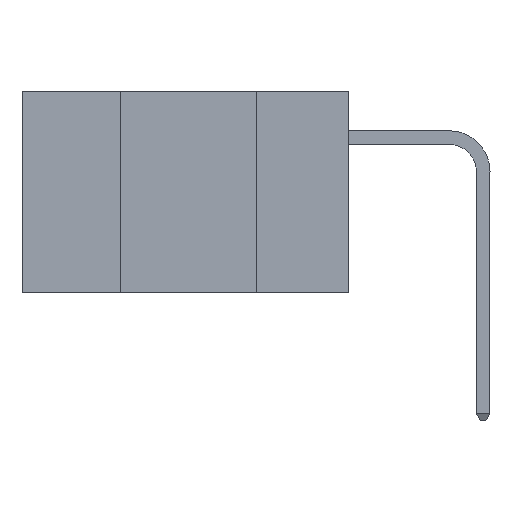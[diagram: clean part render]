
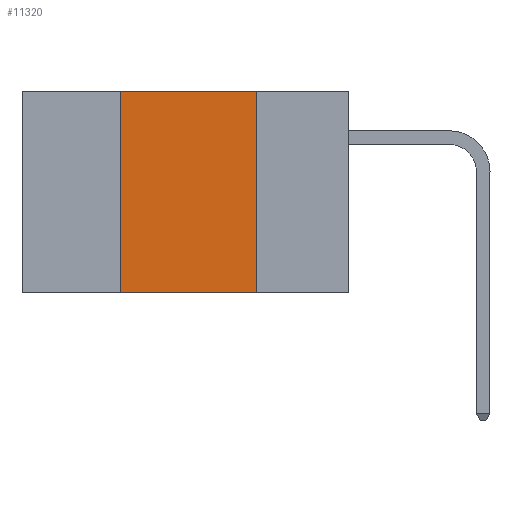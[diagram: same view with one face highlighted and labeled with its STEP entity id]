
A CAD part, left-side view. The second image highlights one B-rep face of the part: STEP entity #11320.
In plain terms, the highlighted planar face has unit normal (-1, 0, 0).
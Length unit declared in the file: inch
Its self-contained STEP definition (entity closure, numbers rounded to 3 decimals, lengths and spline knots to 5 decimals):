
#238 = ORIENTED_EDGE ( 'NONE', *, *, #440, .F. ) ;
#440 = EDGE_CURVE ( 'NONE', #15428, #15209, #568, .T. ) ;
#456 = VERTEX_POINT ( 'NONE', #8224 ) ;
#568 = LINE ( 'NONE', #4432, #764 ) ;
#764 = VECTOR ( 'NONE', #6957, 39.37008 ) ;
#902 = VECTOR ( 'NONE', #11976, 39.37008 ) ;
#975 = ORIENTED_EDGE ( 'NONE', *, *, #14824, .T. ) ;
#1987 = DIRECTION ( 'NONE',  ( 0., 0., -1. ) ) ;
#2430 = ORIENTED_EDGE ( 'NONE', *, *, #14245, .F. ) ;
#4048 = DIRECTION ( 'NONE',  ( 0., 0., 1. ) ) ;
#4276 = CARTESIAN_POINT ( 'NONE',  ( 0., 0.6, -0.37 ) ) ;
#4432 = CARTESIAN_POINT ( 'NONE',  ( 0., 0.6, 0. ) ) ;
#5980 = CARTESIAN_POINT ( 'NONE',  ( 0., 0.42, 0. ) ) ;
#6842 = VERTEX_POINT ( 'NONE', #15889 ) ;
#6936 = PLANE ( 'NONE',  #15651 ) ;
#6957 = DIRECTION ( 'NONE',  ( 0., -1., 0. ) ) ;
#7423 = LINE ( 'NONE', #7819, #14597 ) ;
#7819 = CARTESIAN_POINT ( 'NONE',  ( 0., 0.42, 0. ) ) ;
#8224 = CARTESIAN_POINT ( 'NONE',  ( 0., 0.42, -0.37 ) ) ;
#9269 = LINE ( 'NONE', #14602, #12440 ) ;
#9727 = CARTESIAN_POINT ( 'NONE',  ( 0., 0.6, 0. ) ) ;
#11025 = DIRECTION ( 'NONE',  ( 0., 0., -1. ) ) ;
#11026 = DIRECTION ( 'NONE',  ( 1., 0., 0. ) ) ;
#11164 = ORIENTED_EDGE ( 'NONE', *, *, #15120, .F. ) ;
#11320 = ADVANCED_FACE ( 'NONE', ( #14935 ), #6936, .F. ) ;
#11976 = DIRECTION ( 'NONE',  ( 0., -1., 0. ) ) ;
#12224 = LINE ( 'NONE', #4276, #902 ) ;
#12440 = VECTOR ( 'NONE', #11025, 39.37008 ) ;
#13022 = CARTESIAN_POINT ( 'NONE',  ( 0., 0.17, 0. ) ) ;
#14170 = EDGE_LOOP ( 'NONE', ( #2430, #238, #11164, #975 ) ) ;
#14245 = EDGE_CURVE ( 'NONE', #15209, #6842, #9269, .T. ) ;
#14597 = VECTOR ( 'NONE', #4048, 39.37008 ) ;
#14602 = CARTESIAN_POINT ( 'NONE',  ( 0., 0.17, 0. ) ) ;
#14824 = EDGE_CURVE ( 'NONE', #456, #6842, #12224, .T. ) ;
#14935 = FACE_OUTER_BOUND ( 'NONE', #14170, .T. ) ;
#15120 = EDGE_CURVE ( 'NONE', #456, #15428, #7423, .T. ) ;
#15209 = VERTEX_POINT ( 'NONE', #13022 ) ;
#15428 = VERTEX_POINT ( 'NONE', #5980 ) ;
#15651 = AXIS2_PLACEMENT_3D ( 'NONE', #9727, #11026, #1987 ) ;
#15889 = CARTESIAN_POINT ( 'NONE',  ( 0., 0.17, -0.37 ) ) ;
